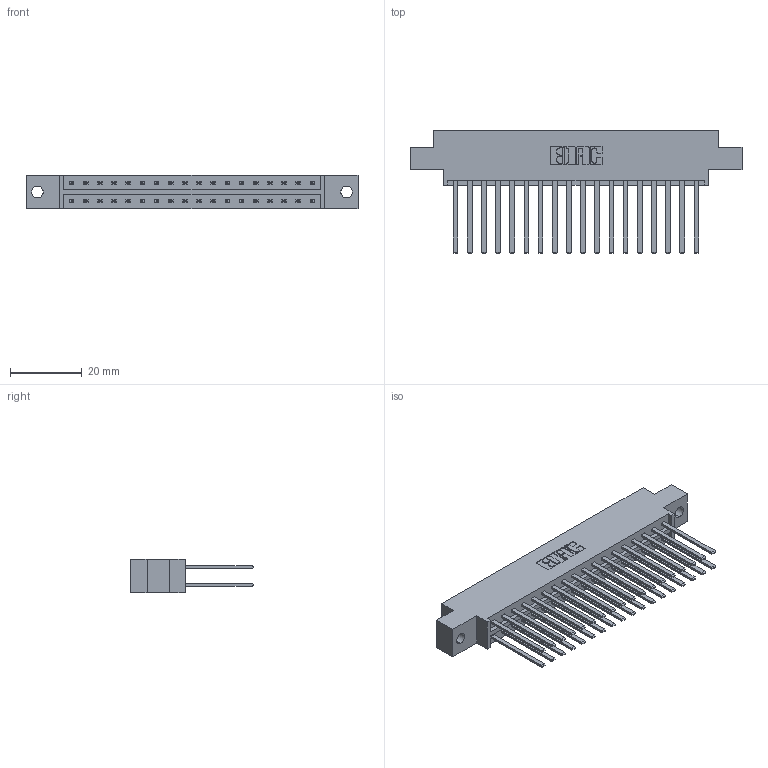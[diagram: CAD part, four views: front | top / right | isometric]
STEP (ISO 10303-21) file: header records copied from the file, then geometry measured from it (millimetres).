
FILE_DESCRIPTION (( 'STEP AP203' ), '1' );
FILE_NAME ('333-036-544-802.STEP', '2018-08-03T01:28:04', ( '' ), ( '' ), 'SwSTEP 2.0', 'SolidWorks 2016', '' );
FILE_SCHEMA (( 'CONFIG_CONTROL_DESIGN' ));
Length unit declared in the file: inch
Products named in the file (3): 333 Part_Offset - .128 Dia; 345-292-001_345-293-144; 333-036-544-802
Assembly tree (37 placements, depth 2):
  333-036-544-802
    333 Part_Offset - .128 Dia
    345-292-001_345-293-144  x36
Bounding box: 92.86 x 34.3 x 9.4 mm (x, y, z)
Volume: 9496.5 mm3; surface area: 12541.6 mm2
Topology: 37 solids, 37 shells, 1774 faces, 5255 edges, 3454 vertices
Faces by surface type: plane 1226, cylinder 548
Entity records: 14635 total; most frequent: CARTESIAN_POINT 2454, ORIENTED_EDGE 2390, DIRECTION 2135, EDGE_CURVE 1195, VECTOR 1071, LINE 1071, VERTEX_POINT 794, AXIS2_PLACEMENT_3D 532
